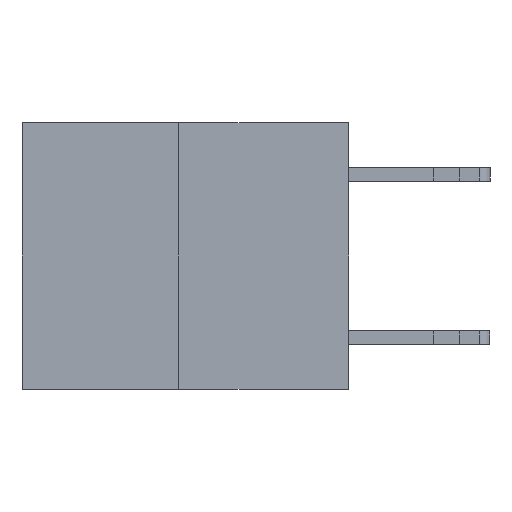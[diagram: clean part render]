
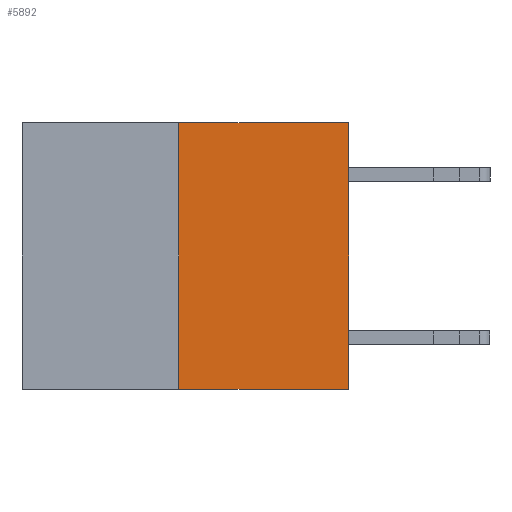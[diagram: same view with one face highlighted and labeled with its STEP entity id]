
A CAD part, left-side view. The second image highlights one B-rep face of the part: STEP entity #5892.
In plain terms, the highlighted planar face has unit normal (-1, 0, 0).
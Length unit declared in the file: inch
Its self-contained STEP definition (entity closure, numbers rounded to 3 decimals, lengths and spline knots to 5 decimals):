
#742 = DIRECTION ( 'NONE',  ( 0., 0., -1. ) ) ;
#1475 = ORIENTED_EDGE ( 'NONE', *, *, #1714, .F. ) ;
#1714 = EDGE_CURVE ( 'NONE', #4871, #12669, #1868, .T. ) ;
#1868 = LINE ( 'NONE', #4943, #14183 ) ;
#2400 = VERTEX_POINT ( 'NONE', #13034 ) ;
#2666 = DIRECTION ( 'NONE',  ( 0., 0., 1. ) ) ;
#3466 = AXIS2_PLACEMENT_3D ( 'NONE', #6526, #4115, #742 ) ;
#4115 = DIRECTION ( 'NONE',  ( 1., 0., 0. ) ) ;
#4236 = EDGE_LOOP ( 'NONE', ( #1475, #9837, #5090, #14577 ) ) ;
#4871 = VERTEX_POINT ( 'NONE', #8648 ) ;
#4943 = CARTESIAN_POINT ( 'NONE',  ( 0., 0.312, -0.49 ) ) ;
#4963 = DIRECTION ( 'NONE',  ( 0., -1., 0. ) ) ;
#5090 = ORIENTED_EDGE ( 'NONE', *, *, #13138, .T. ) ;
#5892 = ADVANCED_FACE ( 'NONE', ( #9011 ), #6485, .F. ) ;
#6485 = PLANE ( 'NONE',  #3466 ) ;
#6526 = CARTESIAN_POINT ( 'NONE',  ( 0., 0.6, 0. ) ) ;
#8186 = CARTESIAN_POINT ( 'NONE',  ( 0., 0.312, 0. ) ) ;
#8242 = CARTESIAN_POINT ( 'NONE',  ( 0., 0.6, -0.49 ) ) ;
#8248 = LINE ( 'NONE', #9451, #12180 ) ;
#8560 = VECTOR ( 'NONE', #9204, 39.37008 ) ;
#8648 = CARTESIAN_POINT ( 'NONE',  ( 0., 0.312, -0.49 ) ) ;
#8912 = CARTESIAN_POINT ( 'NONE',  ( 0., 0., 0. ) ) ;
#9011 = FACE_OUTER_BOUND ( 'NONE', #4236, .T. ) ;
#9204 = DIRECTION ( 'NONE',  ( 0., 0., 1. ) ) ;
#9451 = CARTESIAN_POINT ( 'NONE',  ( 0., 0.6, 0. ) ) ;
#9820 = VERTEX_POINT ( 'NONE', #12393 ) ;
#9837 = ORIENTED_EDGE ( 'NONE', *, *, #11813, .T. ) ;
#9846 = LINE ( 'NONE', #8242, #13060 ) ;
#10491 = DIRECTION ( 'NONE',  ( 0., -1., 0. ) ) ;
#11813 = EDGE_CURVE ( 'NONE', #4871, #9820, #9846, .T. ) ;
#11879 = EDGE_CURVE ( 'NONE', #12669, #2400, #8248, .T. ) ;
#12180 = VECTOR ( 'NONE', #4963, 39.37008 ) ;
#12393 = CARTESIAN_POINT ( 'NONE',  ( 0., 0., -0.49 ) ) ;
#12491 = LINE ( 'NONE', #8912, #8560 ) ;
#12669 = VERTEX_POINT ( 'NONE', #8186 ) ;
#13034 = CARTESIAN_POINT ( 'NONE',  ( 0., 0., 0. ) ) ;
#13060 = VECTOR ( 'NONE', #10491, 39.37008 ) ;
#13138 = EDGE_CURVE ( 'NONE', #9820, #2400, #12491, .T. ) ;
#14183 = VECTOR ( 'NONE', #2666, 39.37008 ) ;
#14577 = ORIENTED_EDGE ( 'NONE', *, *, #11879, .F. ) ;
